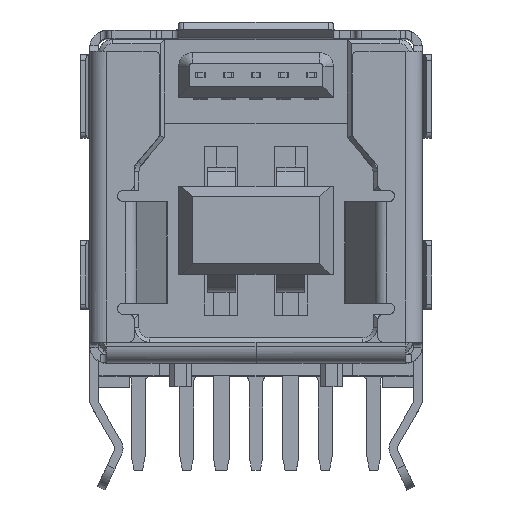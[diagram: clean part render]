
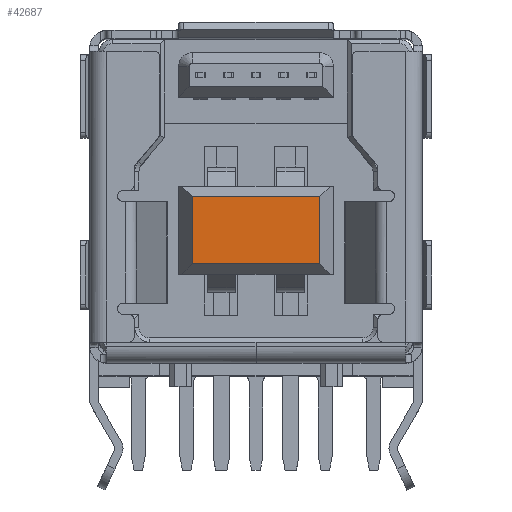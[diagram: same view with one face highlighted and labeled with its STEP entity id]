
A CAD part, top view. The second image highlights one B-rep face of the part: STEP entity #42687.
In plain terms, the highlighted planar face has unit normal (0, 0, 1).
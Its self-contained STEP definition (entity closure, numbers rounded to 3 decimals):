
#30 = DIRECTION ( 'NONE',  ( 0., -1., 0. ) ) ;
#496 = ORIENTED_EDGE ( 'NONE', *, *, #42024, .T. ) ;
#786 = CARTESIAN_POINT ( 'NONE',  ( 2.3, -1.21, -0.5 ) ) ;
#1764 = LINE ( 'NONE', #36170, #10978 ) ;
#2227 = ORIENTED_EDGE ( 'NONE', *, *, #32842, .T. ) ;
#3626 = LINE ( 'NONE', #34547, #42916 ) ;
#6393 = DIRECTION ( 'NONE',  ( -1., 0., 0. ) ) ;
#7051 = VECTOR ( 'NONE', #11157, 1000. ) ;
#8077 = VECTOR ( 'NONE', #30, 1000. ) ;
#9913 = DIRECTION ( 'NONE',  ( 1., 0., 0. ) ) ;
#9983 = ORIENTED_EDGE ( 'NONE', *, *, #20342, .T. ) ;
#10978 = VECTOR ( 'NONE', #15166, 1000. ) ;
#11157 = DIRECTION ( 'NONE',  ( 0., 1., 0. ) ) ;
#11250 = CARTESIAN_POINT ( 'NONE',  ( -2.3, 0., -0.5 ) ) ;
#14035 = ORIENTED_EDGE ( 'NONE', *, *, #33934, .T. ) ;
#14089 = LINE ( 'NONE', #34646, #8077 ) ;
#15166 = DIRECTION ( 'NONE',  ( 1., 0., 0. ) ) ;
#16848 = FACE_OUTER_BOUND ( 'NONE', #43373, .T. ) ;
#17149 = VERTEX_POINT ( 'NONE', #43303 ) ;
#20065 = DIRECTION ( 'NONE',  ( 0., 0., 1. ) ) ;
#20342 = EDGE_CURVE ( 'NONE', #27816, #40009, #3626, .T. ) ;
#23706 = CARTESIAN_POINT ( 'NONE',  ( 2.3, 0., -0.5 ) ) ;
#23976 = PLANE ( 'NONE',  #37278 ) ;
#27816 = VERTEX_POINT ( 'NONE', #23706 ) ;
#30909 = CARTESIAN_POINT ( 'NONE',  ( -2.392, -2.468, -0.5 ) ) ;
#32842 = EDGE_CURVE ( 'NONE', #17149, #37133, #1764, .T. ) ;
#33934 = EDGE_CURVE ( 'NONE', #40009, #17149, #14089, .T. ) ;
#34547 = CARTESIAN_POINT ( 'NONE',  ( 0., 0., -0.5 ) ) ;
#34646 = CARTESIAN_POINT ( 'NONE',  ( -2.3, -1.21, -0.5 ) ) ;
#36170 = CARTESIAN_POINT ( 'NONE',  ( 0., -2.42, -0.5 ) ) ;
#36309 = LINE ( 'NONE', #786, #7051 ) ;
#37133 = VERTEX_POINT ( 'NONE', #42502 ) ;
#37278 = AXIS2_PLACEMENT_3D ( 'NONE', #30909, #20065, #9913 ) ;
#40009 = VERTEX_POINT ( 'NONE', #11250 ) ;
#42024 = EDGE_CURVE ( 'NONE', #37133, #27816, #36309, .T. ) ;
#42502 = CARTESIAN_POINT ( 'NONE',  ( 2.3, -2.42, -0.5 ) ) ;
#42687 = ADVANCED_FACE ( 'NONE', ( #16848 ), #23976, .T. ) ;
#42916 = VECTOR ( 'NONE', #6393, 1000. ) ;
#43303 = CARTESIAN_POINT ( 'NONE',  ( -2.3, -2.42, -0.5 ) ) ;
#43373 = EDGE_LOOP ( 'NONE', ( #14035, #2227, #496, #9983 ) ) ;
